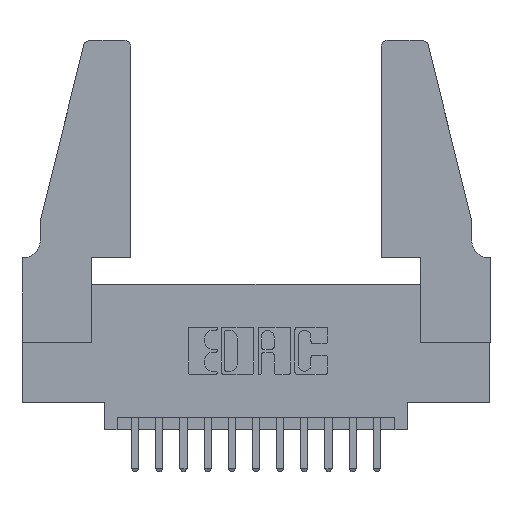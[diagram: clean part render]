
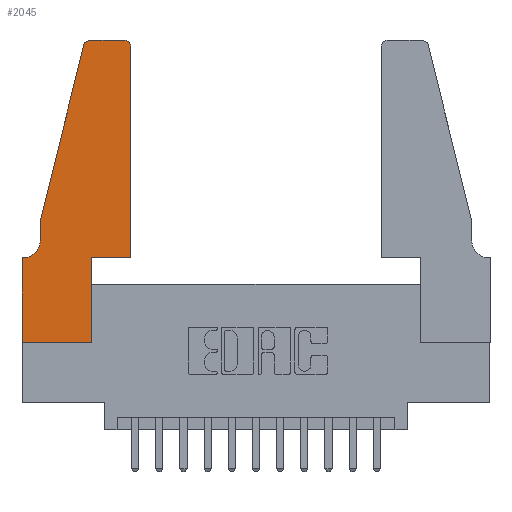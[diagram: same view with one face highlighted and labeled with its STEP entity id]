
A CAD part, top view. The second image highlights one B-rep face of the part: STEP entity #2045.
In plain terms, the highlighted planar face has unit normal (0, 0, 1).
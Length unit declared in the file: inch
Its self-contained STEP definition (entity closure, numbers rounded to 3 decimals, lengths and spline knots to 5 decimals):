
#929 = DIRECTION ( 'NONE',  ( 1., 0., 0. ) ) ;
#1074 = CARTESIAN_POINT ( 'NONE',  ( 0.2865, 0.35, 0.37 ) ) ;
#1432 = LINE ( 'NONE', #6027, #3952 ) ;
#1655 = DIRECTION ( 'NONE',  ( 0., 0., 1. ) ) ;
#2045 = ADVANCED_FACE ( 'NONE', ( #9270 ), #12784, .T. ) ;
#2819 = CARTESIAN_POINT ( 'NONE',  ( 0.2865, 0.35, 0.37 ) ) ;
#3127 = DIRECTION ( 'NONE',  ( -1., 0., 0. ) ) ;
#3303 = ORIENTED_EDGE ( 'NONE', *, *, #6723, .T. ) ;
#3503 = CARTESIAN_POINT ( 'NONE',  ( 0.4505, 1.22, 0.37 ) ) ;
#3860 = DIRECTION ( 'NONE',  ( 0., 0., -1. ) ) ;
#3919 = VERTEX_POINT ( 'NONE', #7676 ) ;
#3952 = VECTOR ( 'NONE', #9532, 39.37008 ) ;
#3984 = CARTESIAN_POINT ( 'NONE',  ( 0.4205, 1.25, 0.37 ) ) ;
#4124 = ORIENTED_EDGE ( 'NONE', *, *, #10493, .T. ) ;
#4281 = EDGE_CURVE ( 'NONE', #8284, #4378, #5252, .T. ) ;
#4378 = VERTEX_POINT ( 'NONE', #3984 ) ;
#4958 = DIRECTION ( 'NONE',  ( 1., 0., 0. ) ) ;
#4960 = CARTESIAN_POINT ( 'NONE',  ( 0.4505, 0.35, 0.37 ) ) ;
#4986 = CARTESIAN_POINT ( 'NONE',  ( 0., 0.35, 0.37 ) ) ;
#4995 = CARTESIAN_POINT ( 'NONE',  ( 0.284, 1.22, 0.37 ) ) ;
#5252 = CIRCLE ( 'NONE', #8250, 0.03 ) ;
#5475 = CARTESIAN_POINT ( 'NONE',  ( 0., 0., 0.37 ) ) ;
#5642 = ORIENTED_EDGE ( 'NONE', *, *, #8734, .T. ) ;
#5979 = VERTEX_POINT ( 'NONE', #13620 ) ;
#6027 = CARTESIAN_POINT ( 'NONE',  ( 0.2605, 1.25, 0.37 ) ) ;
#6042 = CARTESIAN_POINT ( 'NONE',  ( 0.0755, 0.5, 0.37 ) ) ;
#6109 = ORIENTED_EDGE ( 'NONE', *, *, #4281, .T. ) ;
#6135 = DIRECTION ( 'NONE',  ( 0., 1., 0. ) ) ;
#6173 = DIRECTION ( 'NONE',  ( 1., 0., 0. ) ) ;
#6228 = VECTOR ( 'NONE', #10579, 39.37008 ) ;
#6524 = ORIENTED_EDGE ( 'NONE', *, *, #13233, .T. ) ;
#6723 = EDGE_CURVE ( 'NONE', #10957, #11916, #12068, .T. ) ;
#6854 = ORIENTED_EDGE ( 'NONE', *, *, #11863, .T. ) ;
#7059 = VERTEX_POINT ( 'NONE', #5475 ) ;
#7065 = DIRECTION ( 'NONE',  ( 0., 1., 0. ) ) ;
#7082 = DIRECTION ( 'NONE',  ( 1., 0., 0. ) ) ;
#7185 = DIRECTION ( 'NONE',  ( 0., -1., 0. ) ) ;
#7428 = ORIENTED_EDGE ( 'NONE', *, *, #13913, .T. ) ;
#7676 = CARTESIAN_POINT ( 'NONE',  ( 0.2865, 0., 0.37 ) ) ;
#7799 = LINE ( 'NONE', #12653, #13528 ) ;
#8012 = CIRCLE ( 'NONE', #9394, 0.03 ) ;
#8250 = AXIS2_PLACEMENT_3D ( 'NONE', #12846, #14114, #14299 ) ;
#8284 = VERTEX_POINT ( 'NONE', #3503 ) ;
#8370 = DIRECTION ( 'NONE',  ( 0., -1., 0. ) ) ;
#8382 = ORIENTED_EDGE ( 'NONE', *, *, #12286, .T. ) ;
#8668 = CARTESIAN_POINT ( 'NONE',  ( 0.0755, 0.42, 0.37 ) ) ;
#8734 = EDGE_CURVE ( 'NONE', #10573, #10575, #15042, .T. ) ;
#8999 = VECTOR ( 'NONE', #7185, 39.37008 ) ;
#9001 = CARTESIAN_POINT ( 'NONE',  ( 0.0755, 0.5, 0.37 ) ) ;
#9037 = LINE ( 'NONE', #13997, #15121 ) ;
#9084 = EDGE_CURVE ( 'NONE', #11821, #8284, #13076, .T. ) ;
#9262 = LINE ( 'NONE', #15115, #6228 ) ;
#9270 = FACE_OUTER_BOUND ( 'NONE', #15190, .T. ) ;
#9394 = AXIS2_PLACEMENT_3D ( 'NONE', #4995, #13026, #6173 ) ;
#9532 = DIRECTION ( 'NONE',  ( -1., 0., 0. ) ) ;
#10027 = ORIENTED_EDGE ( 'NONE', *, *, #14438, .T. ) ;
#10109 = ORIENTED_EDGE ( 'NONE', *, *, #14327, .T. ) ;
#10127 = LINE ( 'NONE', #15225, #13162 ) ;
#10351 = CARTESIAN_POINT ( 'NONE',  ( 0.284, 1.25, 0.37 ) ) ;
#10493 = EDGE_CURVE ( 'NONE', #5979, #10957, #9262, .T. ) ;
#10572 = ORIENTED_EDGE ( 'NONE', *, *, #9084, .T. ) ;
#10573 = VERTEX_POINT ( 'NONE', #10729 ) ;
#10575 = VERTEX_POINT ( 'NONE', #4986 ) ;
#10579 = DIRECTION ( 'NONE',  ( -0.239, -0.971, 0. ) ) ;
#10729 = CARTESIAN_POINT ( 'NONE',  ( 0.0055, 0.35, 0.37 ) ) ;
#10817 = CARTESIAN_POINT ( 'NONE',  ( 0.0055, 0.42, 0.37 ) ) ;
#10957 = VERTEX_POINT ( 'NONE', #9001 ) ;
#11213 = CIRCLE ( 'NONE', #14194, 0.07 ) ;
#11248 = CARTESIAN_POINT ( 'NONE',  ( 0.0755, 0.35, 0.37 ) ) ;
#11427 = ORIENTED_EDGE ( 'NONE', *, *, #11864, .T. ) ;
#11821 = VERTEX_POINT ( 'NONE', #13990 ) ;
#11863 = EDGE_CURVE ( 'NONE', #10575, #7059, #10127, .T. ) ;
#11864 = EDGE_CURVE ( 'NONE', #4378, #14318, #1432, .T. ) ;
#11916 = VERTEX_POINT ( 'NONE', #8668 ) ;
#11972 = DIRECTION ( 'NONE',  ( -1., 0., 0. ) ) ;
#12027 = VECTOR ( 'NONE', #3127, 39.37008 ) ;
#12068 = LINE ( 'NONE', #6042, #8999 ) ;
#12286 = EDGE_CURVE ( 'NONE', #3919, #13366, #14223, .T. ) ;
#12653 = CARTESIAN_POINT ( 'NONE',  ( 0.4505, 0.35, 0.37 ) ) ;
#12784 = PLANE ( 'NONE',  #13598 ) ;
#12846 = CARTESIAN_POINT ( 'NONE',  ( 0.4205, 1.22, 0.37 ) ) ;
#13026 = DIRECTION ( 'NONE',  ( 0., 0., 1. ) ) ;
#13076 = LINE ( 'NONE', #4960, #13432 ) ;
#13162 = VECTOR ( 'NONE', #8370, 39.37008 ) ;
#13233 = EDGE_CURVE ( 'NONE', #14318, #5979, #8012, .T. ) ;
#13366 = VERTEX_POINT ( 'NONE', #2819 ) ;
#13432 = VECTOR ( 'NONE', #6135, 39.37008 ) ;
#13512 = VECTOR ( 'NONE', #7065, 39.37008 ) ;
#13528 = VECTOR ( 'NONE', #929, 39.37008 ) ;
#13598 = AXIS2_PLACEMENT_3D ( 'NONE', #15131, #1655, #4958 ) ;
#13620 = CARTESIAN_POINT ( 'NONE',  ( 0.25487, 1.22718, 0.37 ) ) ;
#13913 = EDGE_CURVE ( 'NONE', #11916, #10573, #11213, .T. ) ;
#13990 = CARTESIAN_POINT ( 'NONE',  ( 0.4505, 0.35, 0.37 ) ) ;
#13997 = CARTESIAN_POINT ( 'NONE',  ( 0., 0., 0.37 ) ) ;
#14114 = DIRECTION ( 'NONE',  ( 0., 0., 1. ) ) ;
#14194 = AXIS2_PLACEMENT_3D ( 'NONE', #10817, #3860, #11972 ) ;
#14223 = LINE ( 'NONE', #1074, #13512 ) ;
#14299 = DIRECTION ( 'NONE',  ( 1., 0., 0. ) ) ;
#14318 = VERTEX_POINT ( 'NONE', #10351 ) ;
#14327 = EDGE_CURVE ( 'NONE', #13366, #11821, #7799, .T. ) ;
#14438 = EDGE_CURVE ( 'NONE', #7059, #3919, #9037, .T. ) ;
#15042 = LINE ( 'NONE', #11248, #12027 ) ;
#15115 = CARTESIAN_POINT ( 'NONE',  ( 0.0755, 0.5, 0.37 ) ) ;
#15121 = VECTOR ( 'NONE', #7082, 39.37008 ) ;
#15131 = CARTESIAN_POINT ( 'NONE',  ( 0., 0.35, 0.37 ) ) ;
#15190 = EDGE_LOOP ( 'NONE', ( #11427, #6524, #4124, #3303, #7428, #5642, #6854, #10027, #8382, #10109, #10572, #6109 ) ) ;
#15225 = CARTESIAN_POINT ( 'NONE',  ( 0., 0., 0.37 ) ) ;
